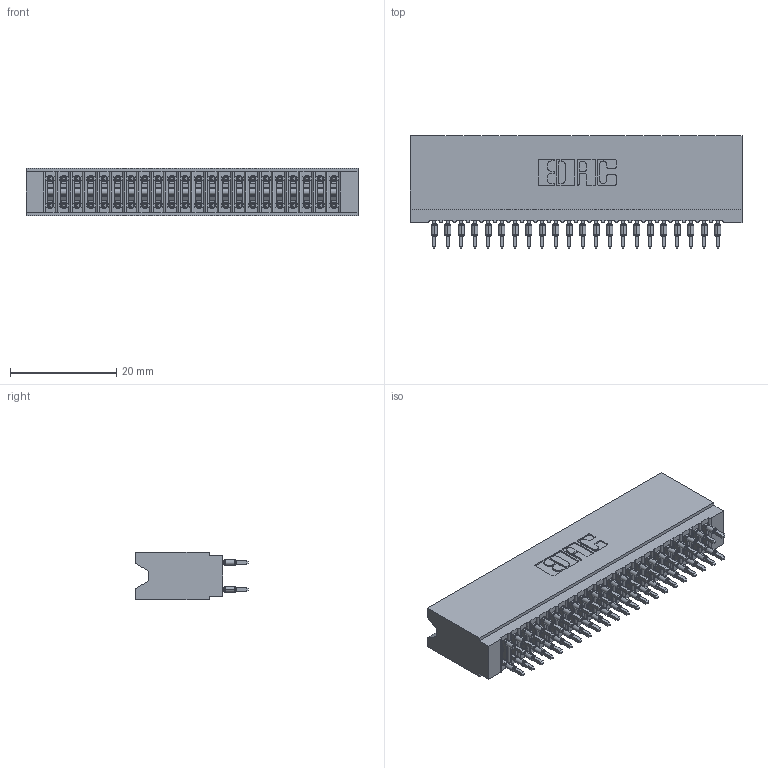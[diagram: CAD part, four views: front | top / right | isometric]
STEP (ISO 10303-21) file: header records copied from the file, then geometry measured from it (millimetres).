
FILE_DESCRIPTION (( 'STEP AP203' ), '1' );
FILE_NAME ('745-044-560-206.STEP', '2026-02-26T17:54:15', ( '' ), ( '' ), 'SwSTEP 2.0', 'SolidWorks 2023', '' );
FILE_SCHEMA (( 'CONFIG_CONTROL_DESIGN' ));
Length unit declared in the file: millimetre
Products named in the file (3): 745-044-560-206; 745-292-001_560; 745 Part_Insulator Option - 06
Assembly tree (45 placements, depth 2):
  745-044-560-206
    745 Part_Insulator Option - 06
    745-292-001_560  x44
Bounding box: 62.48 x 21.22 x 8.89 mm (x, y, z)
Volume: 5888.3 mm3; surface area: 12228.7 mm2
Topology: 45 solids, 45 shells, 4430 faces, 12118 edges, 7696 vertices
Faces by surface type: plane 2300, cylinder 986, bspline 880, torus 264
Entity records: 40111 total; most frequent: CARTESIAN_POINT 7468, ORIENTED_EDGE 6864, DIRECTION 6018, EDGE_CURVE 3432, LINE 3110, VECTOR 3110, VERTEX_POINT 2192, AXIS2_PLACEMENT_3D 1454
